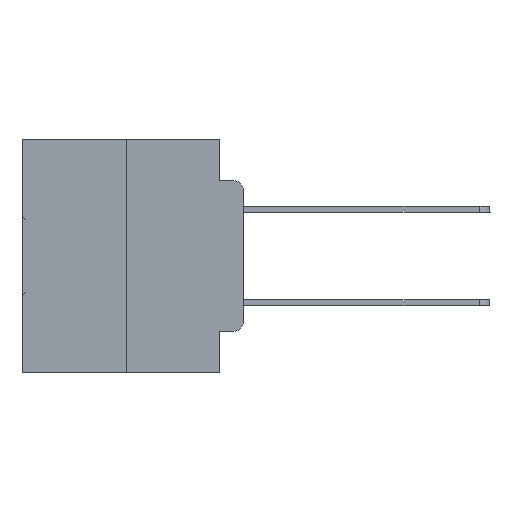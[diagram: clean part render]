
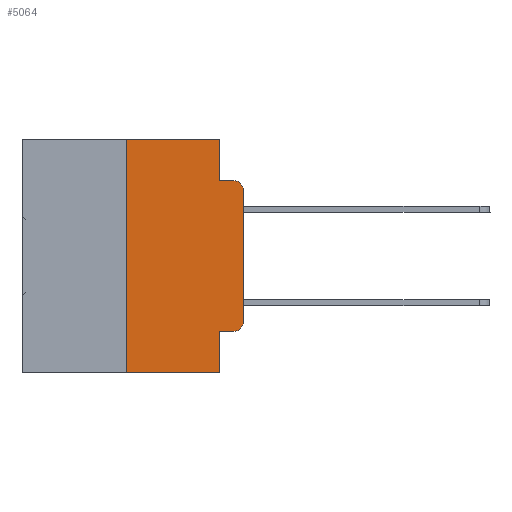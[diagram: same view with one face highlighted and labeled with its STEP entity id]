
A CAD part, left-side view. The second image highlights one B-rep face of the part: STEP entity #5064.
In plain terms, the highlighted planar face has unit normal (-1, 0, 0).
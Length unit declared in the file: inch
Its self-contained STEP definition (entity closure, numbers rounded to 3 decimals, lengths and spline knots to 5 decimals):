
#31 = VECTOR ( 'NONE', #22936, 39.37008 ) ;
#74 = CARTESIAN_POINT ( 'NONE',  ( 0., 0.051, 0. ) ) ;
#223 = AXIS2_PLACEMENT_3D ( 'NONE', #4582, #30233, #7673 ) ;
#274 = VECTOR ( 'NONE', #1678, 39.37008 ) ;
#622 = EDGE_LOOP ( 'NONE', ( #14393, #27758, #14335, #34911, #7812, #34917, #8020, #7739, #2969, #16302 ) ) ;
#1678 = DIRECTION ( 'NONE',  ( 0., -1., 0. ) ) ;
#2346 = VERTEX_POINT ( 'NONE', #11112 ) ;
#2969 = ORIENTED_EDGE ( 'NONE', *, *, #30036, .T. ) ;
#2975 = DIRECTION ( 'NONE',  ( -1., 0., 0. ) ) ;
#3373 = EDGE_CURVE ( 'NONE', #5192, #8761, #14099, .T. ) ;
#3824 = DIRECTION ( 'NONE',  ( 0., -1., 0. ) ) ;
#4582 = CARTESIAN_POINT ( 'NONE',  ( 0., 0.473, 0. ) ) ;
#4607 = EDGE_CURVE ( 'NONE', #8761, #27744, #9984, .T. ) ;
#5064 = ADVANCED_FACE ( 'NONE', ( #10421 ), #10640, .F. ) ;
#5192 = VERTEX_POINT ( 'NONE', #33911 ) ;
#5474 = VECTOR ( 'NONE', #3824, 39.37008 ) ;
#5782 = CARTESIAN_POINT ( 'NONE',  ( 0., 0.25, 0. ) ) ;
#5948 = DIRECTION ( 'NONE',  ( 0., 0., -1. ) ) ;
#7673 = DIRECTION ( 'NONE',  ( 0., 0., -1. ) ) ;
#7739 = ORIENTED_EDGE ( 'NONE', *, *, #16220, .F. ) ;
#7812 = ORIENTED_EDGE ( 'NONE', *, *, #28921, .F. ) ;
#8020 = ORIENTED_EDGE ( 'NONE', *, *, #21182, .T. ) ;
#8235 = VECTOR ( 'NONE', #28208, 39.37008 ) ;
#8350 = VERTEX_POINT ( 'NONE', #14806 ) ;
#8761 = VERTEX_POINT ( 'NONE', #35882 ) ;
#9984 = LINE ( 'NONE', #16916, #8235 ) ;
#10241 = DIRECTION ( 'NONE',  ( 0., -1., 0. ) ) ;
#10421 = FACE_OUTER_BOUND ( 'NONE', #622, .T. ) ;
#10640 = PLANE ( 'NONE',  #223 ) ;
#10994 = VECTOR ( 'NONE', #10241, 39.37008 ) ;
#11112 = CARTESIAN_POINT ( 'NONE',  ( 0., 0.25, 0. ) ) ;
#11504 = CARTESIAN_POINT ( 'NONE',  ( 0., 0., 0. ) ) ;
#11827 = VECTOR ( 'NONE', #33836, 39.37008 ) ;
#12728 = CARTESIAN_POINT ( 'NONE',  ( 0., 0.051, -0.4115 ) ) ;
#12977 = LINE ( 'NONE', #32383, #5474 ) ;
#13537 = EDGE_CURVE ( 'NONE', #22327, #2346, #16391, .T. ) ;
#13683 = LINE ( 'NONE', #24161, #10994 ) ;
#14099 = LINE ( 'NONE', #74, #36487 ) ;
#14260 = EDGE_CURVE ( 'NONE', #19143, #27744, #16823, .T. ) ;
#14320 = DIRECTION ( 'NONE',  ( 0., 0., 1. ) ) ;
#14335 = ORIENTED_EDGE ( 'NONE', *, *, #4607, .F. ) ;
#14393 = ORIENTED_EDGE ( 'NONE', *, *, #33387, .T. ) ;
#14806 = CARTESIAN_POINT ( 'NONE',  ( 0., 0.051, -0.4115 ) ) ;
#16220 = EDGE_CURVE ( 'NONE', #8350, #18866, #35989, .T. ) ;
#16260 = VERTEX_POINT ( 'NONE', #19004 ) ;
#16302 = ORIENTED_EDGE ( 'NONE', *, *, #19784, .T. ) ;
#16391 = LINE ( 'NONE', #5782, #21744 ) ;
#16461 = LINE ( 'NONE', #11504, #31 ) ;
#16823 = CIRCLE ( 'NONE', #31758, 0.02 ) ;
#16916 = CARTESIAN_POINT ( 'NONE',  ( 0., 0.051, -0.0885 ) ) ;
#18227 = DIRECTION ( 'NONE',  ( 0., 0., -1. ) ) ;
#18308 = VERTEX_POINT ( 'NONE', #24411 ) ;
#18866 = VERTEX_POINT ( 'NONE', #35974 ) ;
#19004 = CARTESIAN_POINT ( 'NONE',  ( 0., 0., -0.3915 ) ) ;
#19143 = VERTEX_POINT ( 'NONE', #31811 ) ;
#19784 = EDGE_CURVE ( 'NONE', #18308, #16260, #20905, .T. ) ;
#20131 = CARTESIAN_POINT ( 'NONE',  ( 0., 0.02, -0.1085 ) ) ;
#20905 = CIRCLE ( 'NONE', #23395, 0.02 ) ;
#21182 = EDGE_CURVE ( 'NONE', #22327, #18866, #12977, .T. ) ;
#21483 = CARTESIAN_POINT ( 'NONE',  ( 0., 0.25, -0.5 ) ) ;
#21744 = VECTOR ( 'NONE', #14320, 39.37008 ) ;
#21873 = CARTESIAN_POINT ( 'NONE',  ( 0., 0.051, 0. ) ) ;
#22327 = VERTEX_POINT ( 'NONE', #21483 ) ;
#22936 = DIRECTION ( 'NONE',  ( 0., 0., 1. ) ) ;
#23395 = AXIS2_PLACEMENT_3D ( 'NONE', #32553, #35322, #18227 ) ;
#24161 = CARTESIAN_POINT ( 'NONE',  ( 0., 0.473, 0. ) ) ;
#24411 = CARTESIAN_POINT ( 'NONE',  ( 0., 0.02, -0.4115 ) ) ;
#27744 = VERTEX_POINT ( 'NONE', #31102 ) ;
#27758 = ORIENTED_EDGE ( 'NONE', *, *, #14260, .T. ) ;
#28208 = DIRECTION ( 'NONE',  ( 0., -1., 0. ) ) ;
#28921 = EDGE_CURVE ( 'NONE', #2346, #5192, #13683, .T. ) ;
#30036 = EDGE_CURVE ( 'NONE', #8350, #18308, #36461, .T. ) ;
#30233 = DIRECTION ( 'NONE',  ( 1., 0., 0. ) ) ;
#31102 = CARTESIAN_POINT ( 'NONE',  ( 0., 0.02, -0.0885 ) ) ;
#31758 = AXIS2_PLACEMENT_3D ( 'NONE', #20131, #2975, #31881 ) ;
#31811 = CARTESIAN_POINT ( 'NONE',  ( 0., 0., -0.1085 ) ) ;
#31881 = DIRECTION ( 'NONE',  ( 0., 0., -1. ) ) ;
#32383 = CARTESIAN_POINT ( 'NONE',  ( 0., 0.473, -0.5 ) ) ;
#32553 = CARTESIAN_POINT ( 'NONE',  ( 0., 0.02, -0.3915 ) ) ;
#33387 = EDGE_CURVE ( 'NONE', #16260, #19143, #16461, .T. ) ;
#33836 = DIRECTION ( 'NONE',  ( 0., 0., -1. ) ) ;
#33911 = CARTESIAN_POINT ( 'NONE',  ( 0., 0.051, 0. ) ) ;
#34911 = ORIENTED_EDGE ( 'NONE', *, *, #3373, .F. ) ;
#34917 = ORIENTED_EDGE ( 'NONE', *, *, #13537, .F. ) ;
#35322 = DIRECTION ( 'NONE',  ( -1., 0., 0. ) ) ;
#35882 = CARTESIAN_POINT ( 'NONE',  ( 0., 0.051, -0.0885 ) ) ;
#35974 = CARTESIAN_POINT ( 'NONE',  ( 0., 0.051, -0.5 ) ) ;
#35989 = LINE ( 'NONE', #21873, #11827 ) ;
#36461 = LINE ( 'NONE', #12728, #274 ) ;
#36487 = VECTOR ( 'NONE', #5948, 39.37008 ) ;
